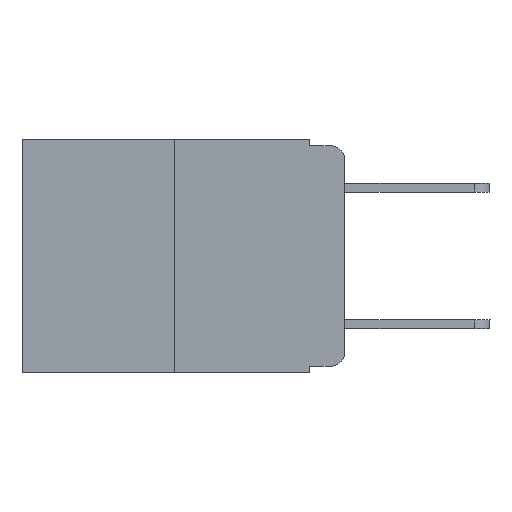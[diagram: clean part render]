
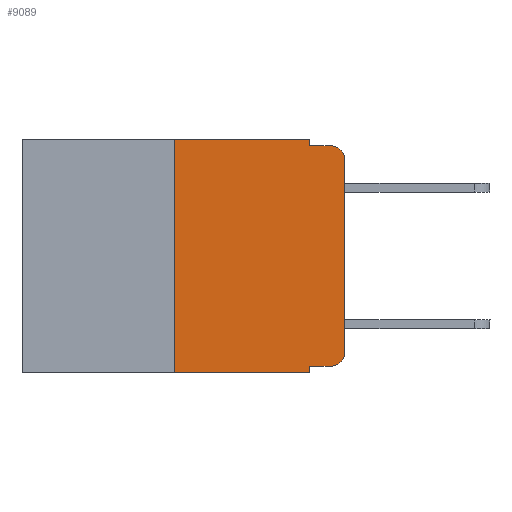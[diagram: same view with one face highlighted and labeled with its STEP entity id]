
A CAD part, left-side view. The second image highlights one B-rep face of the part: STEP entity #9089.
In plain terms, the highlighted planar face has unit normal (-1, 0, 0).
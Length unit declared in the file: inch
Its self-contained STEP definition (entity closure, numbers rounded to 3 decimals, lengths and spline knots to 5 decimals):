
#123 = CARTESIAN_POINT ( 'NONE',  ( 0., 0.051, -0.01 ) ) ;
#320 = PLANE ( 'NONE',  #13990 ) ;
#366 = CARTESIAN_POINT ( 'NONE',  ( 0., 0.02, -0.03 ) ) ;
#508 = ORIENTED_EDGE ( 'NONE', *, *, #1820, .F. ) ;
#520 = CARTESIAN_POINT ( 'NONE',  ( 0., 0.473, 0. ) ) ;
#711 = CARTESIAN_POINT ( 'NONE',  ( 0., 0.25, -0.343 ) ) ;
#787 = VERTEX_POINT ( 'NONE', #711 ) ;
#839 = VERTEX_POINT ( 'NONE', #10349 ) ;
#853 = EDGE_CURVE ( 'NONE', #787, #3259, #2129, .T. ) ;
#881 = DIRECTION ( 'NONE',  ( 0., 0., -1. ) ) ;
#958 = DIRECTION ( 'NONE',  ( 0., 0., 1. ) ) ;
#1142 = EDGE_CURVE ( 'NONE', #839, #5470, #6893, .T. ) ;
#1214 = LINE ( 'NONE', #10691, #12980 ) ;
#1391 = VECTOR ( 'NONE', #881, 39.37008 ) ;
#1534 = DIRECTION ( 'NONE',  ( 0., 0., -1. ) ) ;
#1817 = VECTOR ( 'NONE', #6456, 39.37008 ) ;
#1820 = EDGE_CURVE ( 'NONE', #3259, #839, #2978, .T. ) ;
#1871 = VECTOR ( 'NONE', #958, 39.37008 ) ;
#2129 = LINE ( 'NONE', #12924, #10497 ) ;
#2238 = EDGE_CURVE ( 'NONE', #10218, #7432, #6398, .T. ) ;
#2535 = DIRECTION ( 'NONE',  ( 0., -1., 0. ) ) ;
#2542 = CARTESIAN_POINT ( 'NONE',  ( 0., 0.473, -0.343 ) ) ;
#2727 = CARTESIAN_POINT ( 'NONE',  ( 0., 0.051, -0.343 ) ) ;
#2774 = ORIENTED_EDGE ( 'NONE', *, *, #9882, .F. ) ;
#2882 = LINE ( 'NONE', #11104, #5247 ) ;
#2978 = LINE ( 'NONE', #520, #1817 ) ;
#3050 = ORIENTED_EDGE ( 'NONE', *, *, #2238, .T. ) ;
#3259 = VERTEX_POINT ( 'NONE', #9627 ) ;
#4334 = DIRECTION ( 'NONE',  ( 0., 0., 1. ) ) ;
#4836 = LINE ( 'NONE', #9648, #7769 ) ;
#4932 = ORIENTED_EDGE ( 'NONE', *, *, #8484, .T. ) ;
#5247 = VECTOR ( 'NONE', #14784, 39.37008 ) ;
#5470 = VERTEX_POINT ( 'NONE', #123 ) ;
#5648 = VERTEX_POINT ( 'NONE', #2727 ) ;
#5803 = CARTESIAN_POINT ( 'NONE',  ( 0., 0.051, 0. ) ) ;
#5890 = ORIENTED_EDGE ( 'NONE', *, *, #13500, .T. ) ;
#6196 = CIRCLE ( 'NONE', #8698, 0.02 ) ;
#6310 = VERTEX_POINT ( 'NONE', #11850 ) ;
#6348 = CARTESIAN_POINT ( 'NONE',  ( 0., 0.02, -0.01 ) ) ;
#6398 = CIRCLE ( 'NONE', #6901, 0.02 ) ;
#6413 = LINE ( 'NONE', #2542, #13541 ) ;
#6456 = DIRECTION ( 'NONE',  ( 0., -1., 0. ) ) ;
#6893 = LINE ( 'NONE', #5803, #1391 ) ;
#6901 = AXIS2_PLACEMENT_3D ( 'NONE', #366, #12353, #1534 ) ;
#7153 = ORIENTED_EDGE ( 'NONE', *, *, #853, .F. ) ;
#7319 = DIRECTION ( 'NONE',  ( 0., -1., 0. ) ) ;
#7432 = VERTEX_POINT ( 'NONE', #6348 ) ;
#7641 = CARTESIAN_POINT ( 'NONE',  ( 0., 0., -0.03 ) ) ;
#7769 = VECTOR ( 'NONE', #2535, 39.37008 ) ;
#8073 = CARTESIAN_POINT ( 'NONE',  ( 0., 0., 0. ) ) ;
#8380 = CARTESIAN_POINT ( 'NONE',  ( 0., 0.02, -0.313 ) ) ;
#8484 = EDGE_CURVE ( 'NONE', #13313, #8567, #1214, .T. ) ;
#8567 = VERTEX_POINT ( 'NONE', #13344 ) ;
#8659 = EDGE_LOOP ( 'NONE', ( #5890, #3050, #2774, #13919, #508, #7153, #12081, #11311, #4932, #9314 ) ) ;
#8698 = AXIS2_PLACEMENT_3D ( 'NONE', #8380, #11930, #15280 ) ;
#8852 = FACE_OUTER_BOUND ( 'NONE', #8659, .T. ) ;
#9089 = ADVANCED_FACE ( 'NONE', ( #8852 ), #320, .F. ) ;
#9314 = ORIENTED_EDGE ( 'NONE', *, *, #13442, .T. ) ;
#9627 = CARTESIAN_POINT ( 'NONE',  ( 0., 0.25, 0. ) ) ;
#9648 = CARTESIAN_POINT ( 'NONE',  ( 0., 0.051, -0.01 ) ) ;
#9882 = EDGE_CURVE ( 'NONE', #5470, #7432, #4836, .T. ) ;
#10218 = VERTEX_POINT ( 'NONE', #7641 ) ;
#10229 = EDGE_CURVE ( 'NONE', #13313, #5648, #2882, .T. ) ;
#10349 = CARTESIAN_POINT ( 'NONE',  ( 0., 0.051, 0. ) ) ;
#10497 = VECTOR ( 'NONE', #4334, 39.37008 ) ;
#10556 = CARTESIAN_POINT ( 'NONE',  ( 0., 0.051, -0.333 ) ) ;
#10691 = CARTESIAN_POINT ( 'NONE',  ( 0., 0.051, -0.333 ) ) ;
#11104 = CARTESIAN_POINT ( 'NONE',  ( 0., 0.051, 0. ) ) ;
#11311 = ORIENTED_EDGE ( 'NONE', *, *, #10229, .F. ) ;
#11850 = CARTESIAN_POINT ( 'NONE',  ( 0., 0., -0.313 ) ) ;
#11930 = DIRECTION ( 'NONE',  ( -1., 0., 0. ) ) ;
#12081 = ORIENTED_EDGE ( 'NONE', *, *, #12357, .T. ) ;
#12228 = DIRECTION ( 'NONE',  ( 1., 0., 0. ) ) ;
#12353 = DIRECTION ( 'NONE',  ( -1., 0., 0. ) ) ;
#12357 = EDGE_CURVE ( 'NONE', #787, #5648, #6413, .T. ) ;
#12924 = CARTESIAN_POINT ( 'NONE',  ( 0., 0.25, 0. ) ) ;
#12980 = VECTOR ( 'NONE', #7319, 39.37008 ) ;
#13313 = VERTEX_POINT ( 'NONE', #10556 ) ;
#13344 = CARTESIAN_POINT ( 'NONE',  ( 0., 0.02, -0.333 ) ) ;
#13442 = EDGE_CURVE ( 'NONE', #8567, #6310, #6196, .T. ) ;
#13469 = DIRECTION ( 'NONE',  ( 0., 0., -1. ) ) ;
#13500 = EDGE_CURVE ( 'NONE', #6310, #10218, #14273, .T. ) ;
#13541 = VECTOR ( 'NONE', #14514, 39.37008 ) ;
#13919 = ORIENTED_EDGE ( 'NONE', *, *, #1142, .F. ) ;
#13990 = AXIS2_PLACEMENT_3D ( 'NONE', #14646, #12228, #13469 ) ;
#14273 = LINE ( 'NONE', #8073, #1871 ) ;
#14514 = DIRECTION ( 'NONE',  ( 0., -1., 0. ) ) ;
#14646 = CARTESIAN_POINT ( 'NONE',  ( 0., 0.473, 0. ) ) ;
#14784 = DIRECTION ( 'NONE',  ( 0., 0., -1. ) ) ;
#15280 = DIRECTION ( 'NONE',  ( 0., 0., -1. ) ) ;
